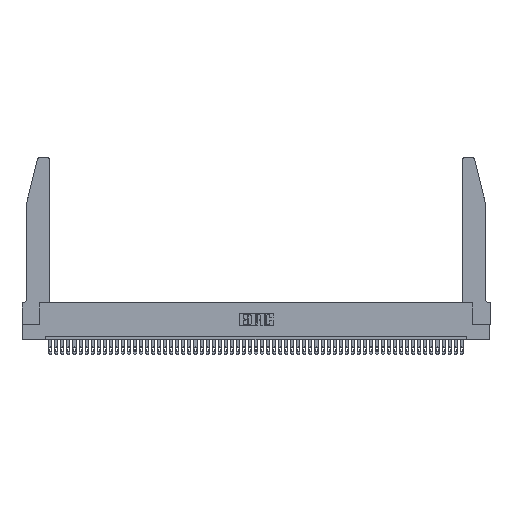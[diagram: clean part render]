
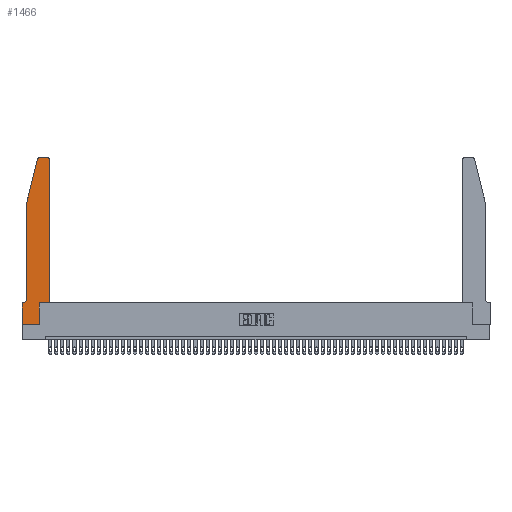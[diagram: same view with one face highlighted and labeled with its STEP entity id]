
A CAD part, top view. The second image highlights one B-rep face of the part: STEP entity #1466.
In plain terms, the highlighted planar face has unit normal (0, 0, 1).
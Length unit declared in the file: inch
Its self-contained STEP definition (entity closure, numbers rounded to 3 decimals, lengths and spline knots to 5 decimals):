
#1225 = CARTESIAN_POINT ( 'NONE',  ( 0.2865, 0.35, 0.37 ) ) ;
#1273 = CARTESIAN_POINT ( 'NONE',  ( 0.0755, 2., 0.37 ) ) ;
#1466 = ADVANCED_FACE ( 'NONE', ( #16070 ), #10517, .T. ) ;
#1656 = CARTESIAN_POINT ( 'NONE',  ( 0.4205, 2.72, 0.37 ) ) ;
#3253 = DIRECTION ( 'NONE',  ( -1., 0., 0. ) ) ;
#3376 = VERTEX_POINT ( 'NONE', #20032 ) ;
#4187 = AXIS2_PLACEMENT_3D ( 'NONE', #22861, #31220, #19268 ) ;
#4744 = EDGE_CURVE ( 'NONE', #43243, #24976, #9996, .T. ) ;
#6269 = ORIENTED_EDGE ( 'NONE', *, *, #18096, .T. ) ;
#6334 = ORIENTED_EDGE ( 'NONE', *, *, #23316, .T. ) ;
#6740 = VERTEX_POINT ( 'NONE', #48911 ) ;
#7033 = LINE ( 'NONE', #30216, #21639 ) ;
#7183 = ORIENTED_EDGE ( 'NONE', *, *, #10075, .T. ) ;
#7620 = VERTEX_POINT ( 'NONE', #10304 ) ;
#7739 = CARTESIAN_POINT ( 'NONE',  ( 0.0755, 2., 0.37 ) ) ;
#7841 = LINE ( 'NONE', #16401, #21149 ) ;
#8308 = VECTOR ( 'NONE', #13607, 39.37008 ) ;
#8349 = ORIENTED_EDGE ( 'NONE', *, *, #8382, .T. ) ;
#8382 = EDGE_CURVE ( 'NONE', #13675, #3376, #7841, .T. ) ;
#9418 = LINE ( 'NONE', #18927, #27538 ) ;
#9902 = DIRECTION ( 'NONE',  ( 1., 0., 0. ) ) ;
#9996 = CIRCLE ( 'NONE', #51963, 0.03 ) ;
#10075 = EDGE_CURVE ( 'NONE', #42462, #43243, #7033, .T. ) ;
#10304 = CARTESIAN_POINT ( 'NONE',  ( 0.2865, 0., 0.37 ) ) ;
#10517 = PLANE ( 'NONE',  #4187 ) ;
#11375 = CIRCLE ( 'NONE', #38219, 0.03 ) ;
#13607 = DIRECTION ( 'NONE',  ( -0.239, -0.971, 0. ) ) ;
#13675 = VERTEX_POINT ( 'NONE', #25732 ) ;
#13793 = DIRECTION ( 'NONE',  ( 0., 0., 1. ) ) ;
#13851 = VERTEX_POINT ( 'NONE', #22489 ) ;
#13871 = EDGE_CURVE ( 'NONE', #28040, #13675, #38005, .T. ) ;
#14351 = VECTOR ( 'NONE', #40629, 39.37008 ) ;
#15146 = VERTEX_POINT ( 'NONE', #24146 ) ;
#16070 = FACE_OUTER_BOUND ( 'NONE', #18132, .T. ) ;
#16091 = CARTESIAN_POINT ( 'NONE',  ( 0., 0., 0.37 ) ) ;
#16401 = CARTESIAN_POINT ( 'NONE',  ( 0.0755, 0.35, 0.37 ) ) ;
#16882 = CARTESIAN_POINT ( 'NONE',  ( 0.0755, 0.42, 0.37 ) ) ;
#17044 = EDGE_CURVE ( 'NONE', #7620, #15146, #22386, .T. ) ;
#18096 = EDGE_CURVE ( 'NONE', #32022, #7620, #9418, .T. ) ;
#18132 = EDGE_LOOP ( 'NONE', ( #7183, #51357, #50595, #21553, #46912, #8349, #23630, #6269, #22381, #6334, #33903, #44410 ) ) ;
#18927 = CARTESIAN_POINT ( 'NONE',  ( 0., 0., 0.37 ) ) ;
#19268 = DIRECTION ( 'NONE',  ( 1., 0., 0. ) ) ;
#19975 = EDGE_CURVE ( 'NONE', #6740, #13851, #20836, .T. ) ;
#20032 = CARTESIAN_POINT ( 'NONE',  ( 0., 0.35, 0.37 ) ) ;
#20836 = LINE ( 'NONE', #45145, #52371 ) ;
#21149 = VECTOR ( 'NONE', #52708, 39.37008 ) ;
#21285 = CARTESIAN_POINT ( 'NONE',  ( 0.25487, 2.72718, 0.37 ) ) ;
#21553 = ORIENTED_EDGE ( 'NONE', *, *, #28926, .T. ) ;
#21639 = VECTOR ( 'NONE', #22021, 39.37008 ) ;
#22021 = DIRECTION ( 'NONE',  ( -1., 0., 0. ) ) ;
#22381 = ORIENTED_EDGE ( 'NONE', *, *, #17044, .T. ) ;
#22386 = LINE ( 'NONE', #1225, #42934 ) ;
#22489 = CARTESIAN_POINT ( 'NONE',  ( 0.4505, 2.72, 0.37 ) ) ;
#22861 = CARTESIAN_POINT ( 'NONE',  ( 0., 0.35, 0.37 ) ) ;
#23316 = EDGE_CURVE ( 'NONE', #15146, #6740, #30438, .T. ) ;
#23470 = DIRECTION ( 'NONE',  ( 1., 0., 0. ) ) ;
#23630 = ORIENTED_EDGE ( 'NONE', *, *, #32222, .T. ) ;
#23974 = CARTESIAN_POINT ( 'NONE',  ( 0.4505, 0.35, 0.37 ) ) ;
#24146 = CARTESIAN_POINT ( 'NONE',  ( 0.2865, 0.35, 0.37 ) ) ;
#24178 = CARTESIAN_POINT ( 'NONE',  ( 0.284, 2.75, 0.37 ) ) ;
#24976 = VERTEX_POINT ( 'NONE', #21285 ) ;
#25732 = CARTESIAN_POINT ( 'NONE',  ( 0.0055, 0.35, 0.37 ) ) ;
#27538 = VECTOR ( 'NONE', #23470, 39.37008 ) ;
#27655 = DIRECTION ( 'NONE',  ( 0., 0., -1. ) ) ;
#28040 = VERTEX_POINT ( 'NONE', #16882 ) ;
#28926 = EDGE_CURVE ( 'NONE', #35795, #28040, #37166, .T. ) ;
#30216 = CARTESIAN_POINT ( 'NONE',  ( 0.2605, 2.75, 0.37 ) ) ;
#30438 = LINE ( 'NONE', #23974, #14351 ) ;
#31220 = DIRECTION ( 'NONE',  ( 0., 0., 1. ) ) ;
#32022 = VERTEX_POINT ( 'NONE', #16091 ) ;
#32222 = EDGE_CURVE ( 'NONE', #3376, #32022, #52499, .T. ) ;
#32367 = CARTESIAN_POINT ( 'NONE',  ( 0.0755, 2., 0.37 ) ) ;
#33636 = AXIS2_PLACEMENT_3D ( 'NONE', #44246, #27655, #3253 ) ;
#33903 = ORIENTED_EDGE ( 'NONE', *, *, #19975, .T. ) ;
#34406 = CARTESIAN_POINT ( 'NONE',  ( 0.4205, 2.75, 0.37 ) ) ;
#34516 = CARTESIAN_POINT ( 'NONE',  ( 0., 0., 0.37 ) ) ;
#35795 = VERTEX_POINT ( 'NONE', #32367 ) ;
#37166 = LINE ( 'NONE', #7739, #43419 ) ;
#38005 = CIRCLE ( 'NONE', #33636, 0.07 ) ;
#38219 = AXIS2_PLACEMENT_3D ( 'NONE', #1656, #38812, #9902 ) ;
#38598 = CARTESIAN_POINT ( 'NONE',  ( 0.284, 2.72, 0.37 ) ) ;
#38812 = DIRECTION ( 'NONE',  ( 0., 0., 1. ) ) ;
#39723 = VECTOR ( 'NONE', #47185, 39.37008 ) ;
#40441 = LINE ( 'NONE', #1273, #8308 ) ;
#40518 = DIRECTION ( 'NONE',  ( 0., -1., 0. ) ) ;
#40629 = DIRECTION ( 'NONE',  ( 1., 0., 0. ) ) ;
#42462 = VERTEX_POINT ( 'NONE', #34406 ) ;
#42666 = DIRECTION ( 'NONE',  ( 1., 0., 0. ) ) ;
#42934 = VECTOR ( 'NONE', #48827, 39.37008 ) ;
#43243 = VERTEX_POINT ( 'NONE', #24178 ) ;
#43419 = VECTOR ( 'NONE', #40518, 39.37008 ) ;
#43823 = EDGE_CURVE ( 'NONE', #13851, #42462, #11375, .T. ) ;
#44246 = CARTESIAN_POINT ( 'NONE',  ( 0.0055, 0.42, 0.37 ) ) ;
#44410 = ORIENTED_EDGE ( 'NONE', *, *, #43823, .T. ) ;
#45145 = CARTESIAN_POINT ( 'NONE',  ( 0.4505, 0.35, 0.37 ) ) ;
#45614 = DIRECTION ( 'NONE',  ( 0., 1., 0. ) ) ;
#46912 = ORIENTED_EDGE ( 'NONE', *, *, #13871, .T. ) ;
#47185 = DIRECTION ( 'NONE',  ( 0., -1., 0. ) ) ;
#47236 = EDGE_CURVE ( 'NONE', #24976, #35795, #40441, .T. ) ;
#48827 = DIRECTION ( 'NONE',  ( 0., 1., 0. ) ) ;
#48911 = CARTESIAN_POINT ( 'NONE',  ( 0.4505, 0.35, 0.37 ) ) ;
#50595 = ORIENTED_EDGE ( 'NONE', *, *, #47236, .T. ) ;
#51357 = ORIENTED_EDGE ( 'NONE', *, *, #4744, .T. ) ;
#51963 = AXIS2_PLACEMENT_3D ( 'NONE', #38598, #13793, #42666 ) ;
#52371 = VECTOR ( 'NONE', #45614, 39.37008 ) ;
#52499 = LINE ( 'NONE', #34516, #39723 ) ;
#52708 = DIRECTION ( 'NONE',  ( -1., 0., 0. ) ) ;
